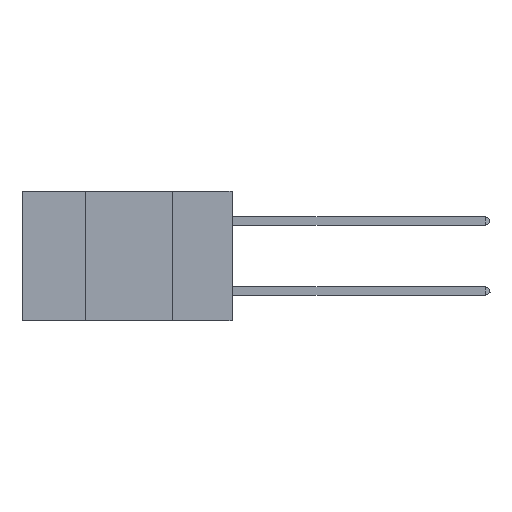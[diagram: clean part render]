
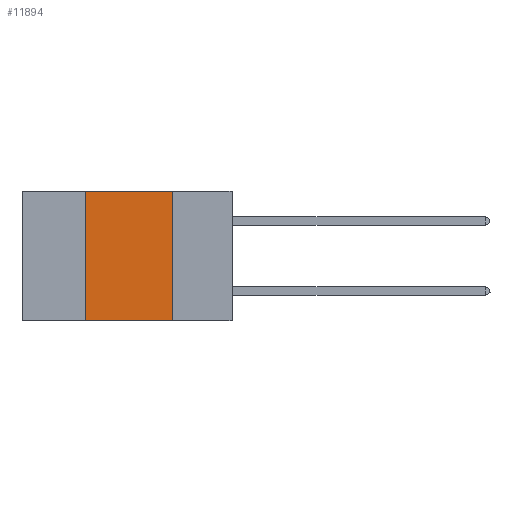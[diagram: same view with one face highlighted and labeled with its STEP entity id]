
A CAD part, left-side view. The second image highlights one B-rep face of the part: STEP entity #11894.
In plain terms, the highlighted planar face has unit normal (-1, 0, 0).
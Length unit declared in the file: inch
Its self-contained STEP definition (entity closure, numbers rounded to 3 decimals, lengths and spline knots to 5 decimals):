
#548 = ORIENTED_EDGE ( 'NONE', *, *, #2587, .T. ) ;
#559 = CARTESIAN_POINT ( 'NONE',  ( 0., 0.6, -0.37 ) ) ;
#621 = DIRECTION ( 'NONE',  ( 1., 0., 0. ) ) ;
#1314 = VECTOR ( 'NONE', #1533, 39.37008 ) ;
#1533 = DIRECTION ( 'NONE',  ( 0., 0., 1. ) ) ;
#1562 = VERTEX_POINT ( 'NONE', #12472 ) ;
#2587 = EDGE_CURVE ( 'NONE', #1562, #7767, #6369, .T. ) ;
#2875 = CARTESIAN_POINT ( 'NONE',  ( 0., 0.42, 0. ) ) ;
#3079 = CARTESIAN_POINT ( 'NONE',  ( 0., 0.6, 0. ) ) ;
#4103 = CARTESIAN_POINT ( 'NONE',  ( 0., 0.17, 0. ) ) ;
#4332 = EDGE_CURVE ( 'NONE', #1562, #17290, #14739, .T. ) ;
#4397 = CARTESIAN_POINT ( 'NONE',  ( 0., 0.17, -0.37 ) ) ;
#4463 = AXIS2_PLACEMENT_3D ( 'NONE', #17949, #621, #16687 ) ;
#5809 = EDGE_CURVE ( 'NONE', #14911, #7767, #5823, .T. ) ;
#5823 = LINE ( 'NONE', #8738, #12204 ) ;
#6114 = LINE ( 'NONE', #3079, #9738 ) ;
#6369 = LINE ( 'NONE', #559, #14573 ) ;
#6453 = PLANE ( 'NONE',  #4463 ) ;
#7767 = VERTEX_POINT ( 'NONE', #4397 ) ;
#8317 = DIRECTION ( 'NONE',  ( 0., 0., -1. ) ) ;
#8738 = CARTESIAN_POINT ( 'NONE',  ( 0., 0.17, 0. ) ) ;
#8840 = DIRECTION ( 'NONE',  ( 0., -1., 0. ) ) ;
#9383 = DIRECTION ( 'NONE',  ( 0., -1., 0. ) ) ;
#9461 = FACE_OUTER_BOUND ( 'NONE', #13784, .T. ) ;
#9738 = VECTOR ( 'NONE', #8840, 39.37008 ) ;
#10371 = EDGE_CURVE ( 'NONE', #17290, #14911, #6114, .T. ) ;
#11894 = ADVANCED_FACE ( 'NONE', ( #9461 ), #6453, .F. ) ;
#12204 = VECTOR ( 'NONE', #8317, 39.37008 ) ;
#12472 = CARTESIAN_POINT ( 'NONE',  ( 0., 0.42, -0.37 ) ) ;
#13784 = EDGE_LOOP ( 'NONE', ( #18778, #17293, #15065, #548 ) ) ;
#14573 = VECTOR ( 'NONE', #9383, 39.37008 ) ;
#14739 = LINE ( 'NONE', #2875, #1314 ) ;
#14911 = VERTEX_POINT ( 'NONE', #4103 ) ;
#15065 = ORIENTED_EDGE ( 'NONE', *, *, #4332, .F. ) ;
#16687 = DIRECTION ( 'NONE',  ( 0., 0., -1. ) ) ;
#17290 = VERTEX_POINT ( 'NONE', #18115 ) ;
#17293 = ORIENTED_EDGE ( 'NONE', *, *, #10371, .F. ) ;
#17949 = CARTESIAN_POINT ( 'NONE',  ( 0., 0.6, 0. ) ) ;
#18115 = CARTESIAN_POINT ( 'NONE',  ( 0., 0.42, 0. ) ) ;
#18778 = ORIENTED_EDGE ( 'NONE', *, *, #5809, .F. ) ;
